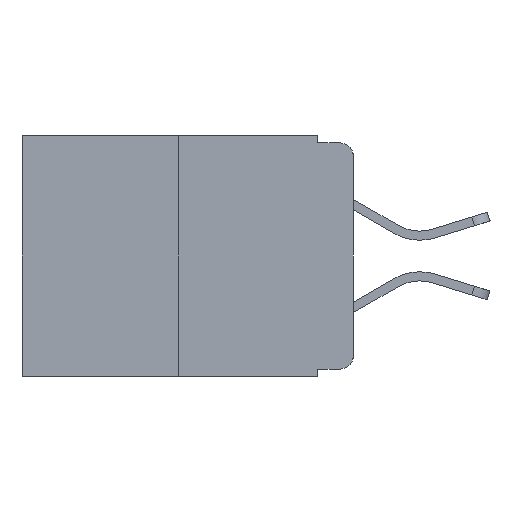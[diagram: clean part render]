
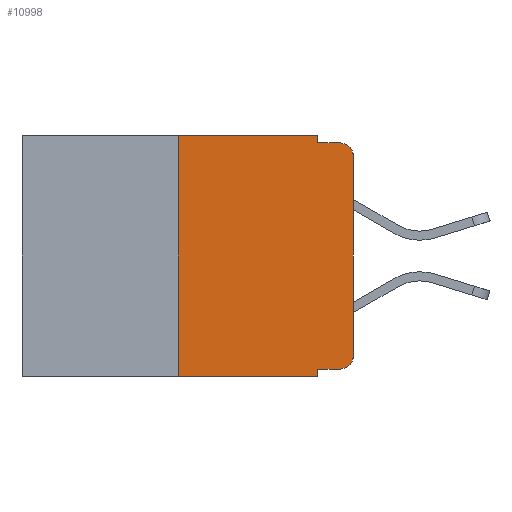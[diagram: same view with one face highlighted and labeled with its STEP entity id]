
A CAD part, left-side view. The second image highlights one B-rep face of the part: STEP entity #10998.
In plain terms, the highlighted planar face has unit normal (-1, 0, 0).
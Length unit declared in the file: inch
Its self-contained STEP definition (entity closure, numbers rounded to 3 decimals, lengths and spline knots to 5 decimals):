
#48 = DIRECTION ( 'NONE',  ( -1., 0., 0. ) ) ;
#282 = CARTESIAN_POINT ( 'NONE',  ( 0., 0.051, 0. ) ) ;
#497 = AXIS2_PLACEMENT_3D ( 'NONE', #9617, #48, #11168 ) ;
#830 = ORIENTED_EDGE ( 'NONE', *, *, #15595, .F. ) ;
#868 = ORIENTED_EDGE ( 'NONE', *, *, #7007, .F. ) ;
#1181 = AXIS2_PLACEMENT_3D ( 'NONE', #7367, #18165, #8989 ) ;
#1443 = ORIENTED_EDGE ( 'NONE', *, *, #5922, .F. ) ;
#1643 = DIRECTION ( 'NONE',  ( 0., 0., -1. ) ) ;
#2335 = CARTESIAN_POINT ( 'NONE',  ( 0., 0.051, -0.333 ) ) ;
#2348 = VERTEX_POINT ( 'NONE', #8185 ) ;
#2497 = CIRCLE ( 'NONE', #1181, 0.02 ) ;
#2515 = EDGE_CURVE ( 'NONE', #13337, #17124, #11710, .T. ) ;
#2711 = ORIENTED_EDGE ( 'NONE', *, *, #2515, .F. ) ;
#2859 = CARTESIAN_POINT ( 'NONE',  ( 0., 0.02, -0.333 ) ) ;
#3853 = EDGE_LOOP ( 'NONE', ( #9244, #4824, #830, #2711, #868, #1443, #5248, #5659, #7417, #12757 ) ) ;
#4095 = DIRECTION ( 'NONE',  ( 0., 0., 1. ) ) ;
#4824 = ORIENTED_EDGE ( 'NONE', *, *, #5340, .T. ) ;
#4978 = CARTESIAN_POINT ( 'NONE',  ( 0., 0.051, -0.343 ) ) ;
#5057 = CARTESIAN_POINT ( 'NONE',  ( 0., 0.051, -0.01 ) ) ;
#5076 = CARTESIAN_POINT ( 'NONE',  ( 0., 0.473, 0. ) ) ;
#5219 = VERTEX_POINT ( 'NONE', #2335 ) ;
#5248 = ORIENTED_EDGE ( 'NONE', *, *, #5347, .T. ) ;
#5256 = CARTESIAN_POINT ( 'NONE',  ( 0., 0., 0. ) ) ;
#5340 = EDGE_CURVE ( 'NONE', #17580, #16316, #2497, .T. ) ;
#5347 = EDGE_CURVE ( 'NONE', #16431, #10437, #18060, .T. ) ;
#5402 = DIRECTION ( 'NONE',  ( 0., 0., 1. ) ) ;
#5627 = DIRECTION ( 'NONE',  ( 0., 0., -1. ) ) ;
#5659 = ORIENTED_EDGE ( 'NONE', *, *, #19263, .F. ) ;
#5922 = EDGE_CURVE ( 'NONE', #16431, #2348, #16150, .T. ) ;
#6168 = DIRECTION ( 'NONE',  ( 0., -1., 0. ) ) ;
#6647 = CARTESIAN_POINT ( 'NONE',  ( 0., 0., -0.03 ) ) ;
#6745 = LINE ( 'NONE', #5076, #14522 ) ;
#6773 = EDGE_CURVE ( 'NONE', #5219, #19504, #7482, .T. ) ;
#6994 = VECTOR ( 'NONE', #6168, 39.37008 ) ;
#7007 = EDGE_CURVE ( 'NONE', #2348, #13337, #6745, .T. ) ;
#7099 = LINE ( 'NONE', #5256, #10778 ) ;
#7367 = CARTESIAN_POINT ( 'NONE',  ( 0., 0.02, -0.03 ) ) ;
#7417 = ORIENTED_EDGE ( 'NONE', *, *, #6773, .T. ) ;
#7482 = LINE ( 'NONE', #17003, #6994 ) ;
#7920 = VECTOR ( 'NONE', #4095, 39.37008 ) ;
#8185 = CARTESIAN_POINT ( 'NONE',  ( 0., 0.25, 0. ) ) ;
#8669 = CARTESIAN_POINT ( 'NONE',  ( 0., 0.051, -0.01 ) ) ;
#8839 = LINE ( 'NONE', #13846, #16535 ) ;
#8989 = DIRECTION ( 'NONE',  ( 0., 0., -1. ) ) ;
#9244 = ORIENTED_EDGE ( 'NONE', *, *, #13914, .T. ) ;
#9312 = LINE ( 'NONE', #5057, #16990 ) ;
#9617 = CARTESIAN_POINT ( 'NONE',  ( 0., 0.02, -0.313 ) ) ;
#10025 = VERTEX_POINT ( 'NONE', #19411 ) ;
#10437 = VERTEX_POINT ( 'NONE', #4978 ) ;
#10537 = DIRECTION ( 'NONE',  ( 0., -1., 0. ) ) ;
#10778 = VECTOR ( 'NONE', #5402, 39.37008 ) ;
#10998 = ADVANCED_FACE ( 'NONE', ( #12931 ), #18718, .F. ) ;
#11105 = DIRECTION ( 'NONE',  ( 1., 0., 0. ) ) ;
#11168 = DIRECTION ( 'NONE',  ( 0., 0., -1. ) ) ;
#11710 = LINE ( 'NONE', #282, #19327 ) ;
#12757 = ORIENTED_EDGE ( 'NONE', *, *, #14892, .T. ) ;
#12909 = CARTESIAN_POINT ( 'NONE',  ( 0., 0.25, -0.343 ) ) ;
#12931 = FACE_OUTER_BOUND ( 'NONE', #3853, .T. ) ;
#13059 = CARTESIAN_POINT ( 'NONE',  ( 0., 0.02, -0.01 ) ) ;
#13337 = VERTEX_POINT ( 'NONE', #18503 ) ;
#13846 = CARTESIAN_POINT ( 'NONE',  ( 0., 0.051, 0. ) ) ;
#13914 = EDGE_CURVE ( 'NONE', #10025, #17580, #7099, .T. ) ;
#14008 = VECTOR ( 'NONE', #10537, 39.37008 ) ;
#14486 = CARTESIAN_POINT ( 'NONE',  ( 0., 0.473, 0. ) ) ;
#14513 = DIRECTION ( 'NONE',  ( 0., -1., 0. ) ) ;
#14522 = VECTOR ( 'NONE', #14513, 39.37008 ) ;
#14892 = EDGE_CURVE ( 'NONE', #19504, #10025, #18195, .T. ) ;
#15103 = CARTESIAN_POINT ( 'NONE',  ( 0., 0.473, -0.343 ) ) ;
#15595 = EDGE_CURVE ( 'NONE', #17124, #16316, #9312, .T. ) ;
#16150 = LINE ( 'NONE', #17954, #7920 ) ;
#16226 = DIRECTION ( 'NONE',  ( 0., 0., -1. ) ) ;
#16316 = VERTEX_POINT ( 'NONE', #13059 ) ;
#16431 = VERTEX_POINT ( 'NONE', #12909 ) ;
#16535 = VECTOR ( 'NONE', #16226, 39.37008 ) ;
#16990 = VECTOR ( 'NONE', #17444, 39.37008 ) ;
#17003 = CARTESIAN_POINT ( 'NONE',  ( 0., 0.051, -0.333 ) ) ;
#17124 = VERTEX_POINT ( 'NONE', #8669 ) ;
#17444 = DIRECTION ( 'NONE',  ( 0., -1., 0. ) ) ;
#17580 = VERTEX_POINT ( 'NONE', #6647 ) ;
#17954 = CARTESIAN_POINT ( 'NONE',  ( 0., 0.25, 0. ) ) ;
#18060 = LINE ( 'NONE', #15103, #14008 ) ;
#18165 = DIRECTION ( 'NONE',  ( -1., 0., 0. ) ) ;
#18195 = CIRCLE ( 'NONE', #497, 0.02 ) ;
#18227 = AXIS2_PLACEMENT_3D ( 'NONE', #14486, #11105, #1643 ) ;
#18503 = CARTESIAN_POINT ( 'NONE',  ( 0., 0.051, 0. ) ) ;
#18718 = PLANE ( 'NONE',  #18227 ) ;
#19263 = EDGE_CURVE ( 'NONE', #5219, #10437, #8839, .T. ) ;
#19327 = VECTOR ( 'NONE', #5627, 39.37008 ) ;
#19411 = CARTESIAN_POINT ( 'NONE',  ( 0., 0., -0.313 ) ) ;
#19504 = VERTEX_POINT ( 'NONE', #2859 ) ;
